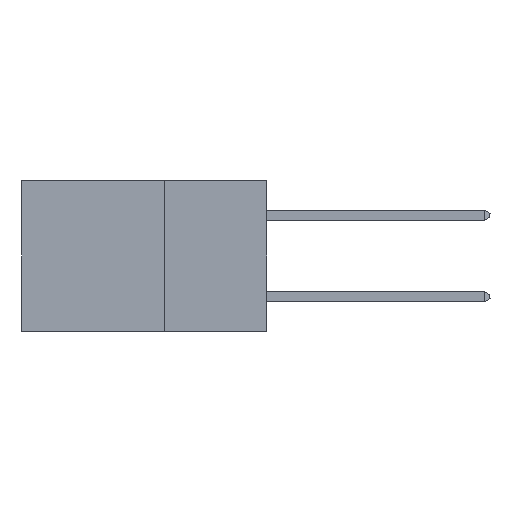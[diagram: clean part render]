
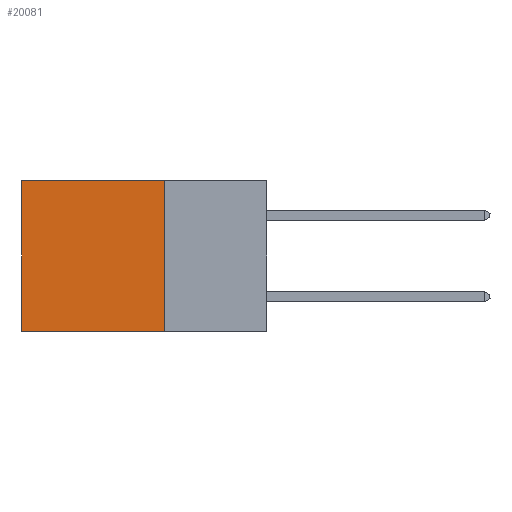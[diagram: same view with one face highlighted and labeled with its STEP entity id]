
A CAD part, left-side view. The second image highlights one B-rep face of the part: STEP entity #20081.
In plain terms, the highlighted planar face has unit normal (-1, 0, 0).
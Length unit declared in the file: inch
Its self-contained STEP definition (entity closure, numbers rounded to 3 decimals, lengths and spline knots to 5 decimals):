
#484 = DIRECTION ( 'NONE',  ( 0., 1., 0. ) ) ;
#1300 = DIRECTION ( 'NONE',  ( 0., 0., -1. ) ) ;
#1895 = CARTESIAN_POINT ( 'NONE',  ( 0.2875, 0.25, -0.37 ) ) ;
#1956 = ORIENTED_EDGE ( 'NONE', *, *, #11315, .T. ) ;
#2109 = CARTESIAN_POINT ( 'NONE',  ( 0.2875, 0.6, -0.37 ) ) ;
#3662 = ORIENTED_EDGE ( 'NONE', *, *, #25561, .F. ) ;
#3718 = VECTOR ( 'NONE', #29421, 39.37008 ) ;
#5269 = PLANE ( 'NONE',  #12370 ) ;
#5608 = DIRECTION ( 'NONE',  ( 0., 1., 0. ) ) ;
#5696 = FACE_OUTER_BOUND ( 'NONE', #23379, .T. ) ;
#7220 = CARTESIAN_POINT ( 'NONE',  ( 0.2875, 0.25, 0. ) ) ;
#7864 = VERTEX_POINT ( 'NONE', #7220 ) ;
#8339 = CARTESIAN_POINT ( 'NONE',  ( 0.2875, 0.25, 0. ) ) ;
#10345 = CARTESIAN_POINT ( 'NONE',  ( 0.2875, 0.25, 0. ) ) ;
#11315 = EDGE_CURVE ( 'NONE', #7864, #29242, #21714, .T. ) ;
#12370 = AXIS2_PLACEMENT_3D ( 'NONE', #31553, #13506, #21366 ) ;
#13038 = VECTOR ( 'NONE', #1300, 39.37008 ) ;
#13298 = CARTESIAN_POINT ( 'NONE',  ( 0.2875, 0.25, -0.37 ) ) ;
#13506 = DIRECTION ( 'NONE',  ( 1., 0., 0. ) ) ;
#14442 = ORIENTED_EDGE ( 'NONE', *, *, #27715, .T. ) ;
#14996 = VERTEX_POINT ( 'NONE', #2109 ) ;
#18982 = CARTESIAN_POINT ( 'NONE',  ( 0.2875, 0.6, 0. ) ) ;
#20081 = ADVANCED_FACE ( 'NONE', ( #5696 ), #5269, .F. ) ;
#21118 = LINE ( 'NONE', #10345, #3718 ) ;
#21366 = DIRECTION ( 'NONE',  ( 0., 0., -1. ) ) ;
#21714 = LINE ( 'NONE', #8339, #33324 ) ;
#23379 = EDGE_LOOP ( 'NONE', ( #14442, #32496, #3662, #1956 ) ) ;
#23591 = VERTEX_POINT ( 'NONE', #1895 ) ;
#24321 = LINE ( 'NONE', #13298, #24771 ) ;
#24771 = VECTOR ( 'NONE', #5608, 39.37008 ) ;
#25561 = EDGE_CURVE ( 'NONE', #7864, #23591, #21118, .T. ) ;
#27121 = LINE ( 'NONE', #30911, #13038 ) ;
#27715 = EDGE_CURVE ( 'NONE', #29242, #14996, #27121, .T. ) ;
#29242 = VERTEX_POINT ( 'NONE', #18982 ) ;
#29421 = DIRECTION ( 'NONE',  ( 0., 0., -1. ) ) ;
#30911 = CARTESIAN_POINT ( 'NONE',  ( 0.2875, 0.6, 0. ) ) ;
#31553 = CARTESIAN_POINT ( 'NONE',  ( 0.2875, 0.25, 0. ) ) ;
#32496 = ORIENTED_EDGE ( 'NONE', *, *, #34243, .F. ) ;
#33324 = VECTOR ( 'NONE', #484, 39.37008 ) ;
#34243 = EDGE_CURVE ( 'NONE', #23591, #14996, #24321, .T. ) ;
